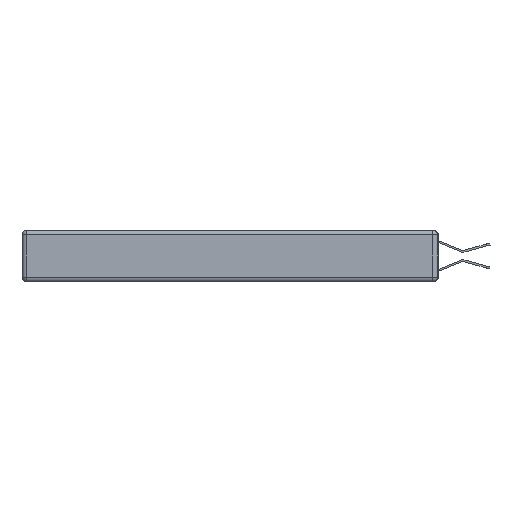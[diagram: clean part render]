
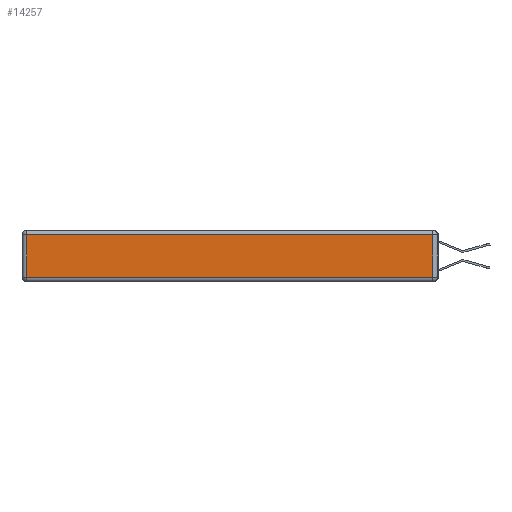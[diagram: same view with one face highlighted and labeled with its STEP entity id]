
A CAD part, left-side view. The second image highlights one B-rep face of the part: STEP entity #14257.
In plain terms, the highlighted planar face has unit normal (-1, 0, 0).
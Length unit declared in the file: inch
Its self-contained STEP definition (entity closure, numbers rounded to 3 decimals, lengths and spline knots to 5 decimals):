
#44 = VERTEX_POINT ( 'NONE', #4765 ) ;
#1481 = VERTEX_POINT ( 'NONE', #26330 ) ;
#1974 = CARTESIAN_POINT ( 'NONE',  ( 0., 2.75, -0.03 ) ) ;
#2740 = CARTESIAN_POINT ( 'NONE',  ( 0., 2.72, -0.03 ) ) ;
#2790 = FACE_OUTER_BOUND ( 'NONE', #17131, .T. ) ;
#3247 = CARTESIAN_POINT ( 'NONE',  ( 0., 0., -0.313 ) ) ;
#3504 = AXIS2_PLACEMENT_3D ( 'NONE', #7958, #22365, #7766 ) ;
#4096 = ORIENTED_EDGE ( 'NONE', *, *, #13158, .T. ) ;
#4765 = CARTESIAN_POINT ( 'NONE',  ( 0., 0.03, -0.313 ) ) ;
#6367 = LINE ( 'NONE', #1974, #26675 ) ;
#6643 = CARTESIAN_POINT ( 'NONE',  ( 0., 0.03, -0.343 ) ) ;
#6759 = EDGE_CURVE ( 'NONE', #15630, #44, #22972, .T. ) ;
#7105 = ORIENTED_EDGE ( 'NONE', *, *, #6759, .T. ) ;
#7766 = DIRECTION ( 'NONE',  ( 0., 0., 1. ) ) ;
#7812 = LINE ( 'NONE', #16842, #11783 ) ;
#7958 = CARTESIAN_POINT ( 'NONE',  ( 0., 0., -0.343 ) ) ;
#8378 = DIRECTION ( 'NONE',  ( 0., 0., -1. ) ) ;
#9594 = EDGE_CURVE ( 'NONE', #1481, #24626, #6367, .T. ) ;
#10664 = DIRECTION ( 'NONE',  ( 0., 1., 0. ) ) ;
#10670 = EDGE_CURVE ( 'NONE', #44, #1481, #18805, .T. ) ;
#11643 = DIRECTION ( 'NONE',  ( 0., -1., 0. ) ) ;
#11783 = VECTOR ( 'NONE', #8378, 39.37008 ) ;
#13158 = EDGE_CURVE ( 'NONE', #24626, #15630, #7812, .T. ) ;
#14257 = ADVANCED_FACE ( 'NONE', ( #2790 ), #16058, .T. ) ;
#15630 = VERTEX_POINT ( 'NONE', #20490 ) ;
#16058 = PLANE ( 'NONE',  #3504 ) ;
#16842 = CARTESIAN_POINT ( 'NONE',  ( 0., 2.72, -0.343 ) ) ;
#17131 = EDGE_LOOP ( 'NONE', ( #7105, #17791, #27027, #4096 ) ) ;
#17791 = ORIENTED_EDGE ( 'NONE', *, *, #10670, .T. ) ;
#18805 = LINE ( 'NONE', #6643, #25316 ) ;
#19400 = VECTOR ( 'NONE', #11643, 39.37008 ) ;
#20490 = CARTESIAN_POINT ( 'NONE',  ( 0., 2.72, -0.313 ) ) ;
#22365 = DIRECTION ( 'NONE',  ( -1., 0., 0. ) ) ;
#22972 = LINE ( 'NONE', #3247, #19400 ) ;
#24626 = VERTEX_POINT ( 'NONE', #2740 ) ;
#25241 = DIRECTION ( 'NONE',  ( 0., 0., 1. ) ) ;
#25316 = VECTOR ( 'NONE', #25241, 39.37008 ) ;
#26330 = CARTESIAN_POINT ( 'NONE',  ( 0., 0.03, -0.03 ) ) ;
#26675 = VECTOR ( 'NONE', #10664, 39.37008 ) ;
#27027 = ORIENTED_EDGE ( 'NONE', *, *, #9594, .T. ) ;
